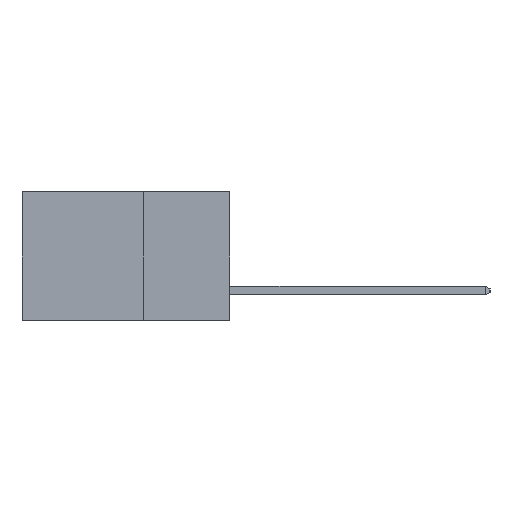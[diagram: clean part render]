
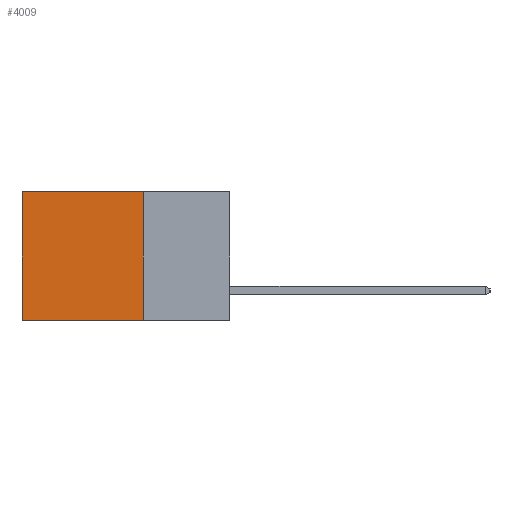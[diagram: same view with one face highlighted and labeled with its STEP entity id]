
A CAD part, left-side view. The second image highlights one B-rep face of the part: STEP entity #4009.
In plain terms, the highlighted planar face has unit normal (-1, 0, 0).
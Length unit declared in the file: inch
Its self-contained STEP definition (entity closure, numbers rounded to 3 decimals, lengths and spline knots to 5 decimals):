
#1793 = VECTOR ( 'NONE', #2302, 39.37008 ) ;
#2302 = DIRECTION ( 'NONE',  ( 0., 1., 0. ) ) ;
#2736 = CARTESIAN_POINT ( 'NONE',  ( 0.2615, 0.25, -0.37 ) ) ;
#3538 = EDGE_CURVE ( 'NONE', #5389, #22526, #10183, .T. ) ;
#4009 = ADVANCED_FACE ( 'NONE', ( #13271 ), #11058, .F. ) ;
#4305 = EDGE_CURVE ( 'NONE', #14497, #22526, #20573, .T. ) ;
#5389 = VERTEX_POINT ( 'NONE', #12568 ) ;
#5597 = VECTOR ( 'NONE', #21562, 39.37008 ) ;
#6279 = ORIENTED_EDGE ( 'NONE', *, *, #3538, .T. ) ;
#6612 = AXIS2_PLACEMENT_3D ( 'NONE', #11678, #10954, #10936 ) ;
#8968 = CARTESIAN_POINT ( 'NONE',  ( 0.2615, 0.25, 0. ) ) ;
#9212 = ORIENTED_EDGE ( 'NONE', *, *, #4305, .F. ) ;
#10183 = LINE ( 'NONE', #19431, #19049 ) ;
#10936 = DIRECTION ( 'NONE',  ( 0., 0., -1. ) ) ;
#10954 = DIRECTION ( 'NONE',  ( 1., 0., 0. ) ) ;
#11032 = ORIENTED_EDGE ( 'NONE', *, *, #17585, .T. ) ;
#11056 = EDGE_LOOP ( 'NONE', ( #6279, #9212, #19843, #11032 ) ) ;
#11058 = PLANE ( 'NONE',  #6612 ) ;
#11678 = CARTESIAN_POINT ( 'NONE',  ( 0.2615, 0.25, -0.37 ) ) ;
#12207 = CARTESIAN_POINT ( 'NONE',  ( 0.2615, 0.25, -0.37 ) ) ;
#12568 = CARTESIAN_POINT ( 'NONE',  ( 0.2615, 0.6, 0. ) ) ;
#13271 = FACE_OUTER_BOUND ( 'NONE', #11056, .T. ) ;
#14158 = EDGE_CURVE ( 'NONE', #18379, #14497, #15105, .T. ) ;
#14336 = DIRECTION ( 'NONE',  ( 0., 1., 0. ) ) ;
#14497 = VERTEX_POINT ( 'NONE', #12207 ) ;
#15105 = LINE ( 'NONE', #19862, #5597 ) ;
#16531 = CARTESIAN_POINT ( 'NONE',  ( 0.2615, 0.25, 0. ) ) ;
#16738 = CARTESIAN_POINT ( 'NONE',  ( 0.2615, 0.6, -0.37 ) ) ;
#17585 = EDGE_CURVE ( 'NONE', #18379, #5389, #19301, .T. ) ;
#18379 = VERTEX_POINT ( 'NONE', #16531 ) ;
#19049 = VECTOR ( 'NONE', #20202, 39.37008 ) ;
#19301 = LINE ( 'NONE', #8968, #21963 ) ;
#19431 = CARTESIAN_POINT ( 'NONE',  ( 0.2615, 0.6, -0.37 ) ) ;
#19843 = ORIENTED_EDGE ( 'NONE', *, *, #14158, .F. ) ;
#19862 = CARTESIAN_POINT ( 'NONE',  ( 0.2615, 0.25, -0.37 ) ) ;
#20202 = DIRECTION ( 'NONE',  ( 0., 0., -1. ) ) ;
#20573 = LINE ( 'NONE', #2736, #1793 ) ;
#21562 = DIRECTION ( 'NONE',  ( 0., 0., -1. ) ) ;
#21963 = VECTOR ( 'NONE', #14336, 39.37008 ) ;
#22526 = VERTEX_POINT ( 'NONE', #16738 ) ;
